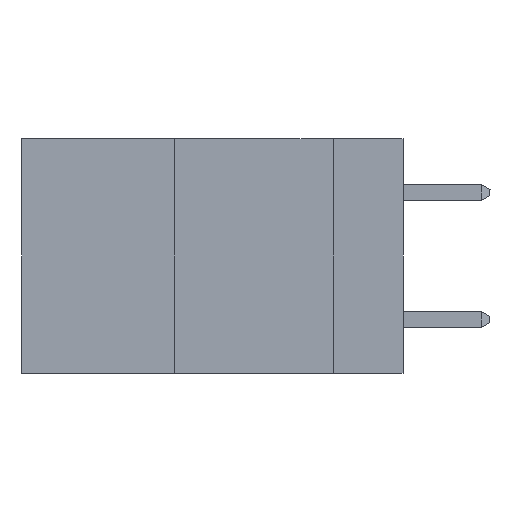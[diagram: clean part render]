
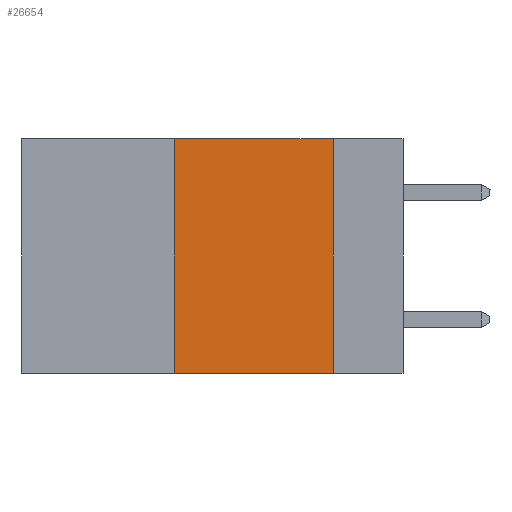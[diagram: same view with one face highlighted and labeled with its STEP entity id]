
A CAD part, left-side view. The second image highlights one B-rep face of the part: STEP entity #26654.
In plain terms, the highlighted planar face has unit normal (-1, 0, 0).
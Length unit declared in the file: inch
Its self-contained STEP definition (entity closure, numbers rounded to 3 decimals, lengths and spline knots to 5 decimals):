
#733 = VERTEX_POINT ( 'NONE', #2641 ) ;
#1047 = VECTOR ( 'NONE', #27830, 39.37008 ) ;
#1316 = VECTOR ( 'NONE', #24645, 39.37008 ) ;
#1868 = EDGE_LOOP ( 'NONE', ( #24799, #25606, #3925, #4275 ) ) ;
#2158 = EDGE_CURVE ( 'NONE', #22826, #16824, #6789, .T. ) ;
#2383 = LINE ( 'NONE', #14751, #27492 ) ;
#2428 = CARTESIAN_POINT ( 'NONE',  ( 0., 0.36, 0. ) ) ;
#2641 = CARTESIAN_POINT ( 'NONE',  ( 0., 0.11, -0.37 ) ) ;
#3925 = ORIENTED_EDGE ( 'NONE', *, *, #2158, .F. ) ;
#3987 = DIRECTION ( 'NONE',  ( 0., -1., 0. ) ) ;
#4230 = PLANE ( 'NONE',  #8082 ) ;
#4275 = ORIENTED_EDGE ( 'NONE', *, *, #17643, .T. ) ;
#4568 = DIRECTION ( 'NONE',  ( 0., 0., -1. ) ) ;
#4809 = CARTESIAN_POINT ( 'NONE',  ( 0., 0.11, 0. ) ) ;
#6434 = VERTEX_POINT ( 'NONE', #4809 ) ;
#6624 = CARTESIAN_POINT ( 'NONE',  ( 0., 0.11, 0. ) ) ;
#6789 = LINE ( 'NONE', #2428, #1047 ) ;
#7652 = EDGE_CURVE ( 'NONE', #16824, #6434, #24380, .T. ) ;
#8082 = AXIS2_PLACEMENT_3D ( 'NONE', #21525, #8178, #21116 ) ;
#8178 = DIRECTION ( 'NONE',  ( 1., 0., 0. ) ) ;
#9931 = CARTESIAN_POINT ( 'NONE',  ( 0., 0.36, 0. ) ) ;
#11868 = VECTOR ( 'NONE', #4568, 39.37008 ) ;
#14074 = CARTESIAN_POINT ( 'NONE',  ( 0., 0.6, 0. ) ) ;
#14751 = CARTESIAN_POINT ( 'NONE',  ( 0., 0.6, -0.37 ) ) ;
#16824 = VERTEX_POINT ( 'NONE', #9931 ) ;
#17123 = EDGE_CURVE ( 'NONE', #6434, #733, #17613, .T. ) ;
#17613 = LINE ( 'NONE', #6624, #11868 ) ;
#17643 = EDGE_CURVE ( 'NONE', #22826, #733, #2383, .T. ) ;
#21116 = DIRECTION ( 'NONE',  ( 0., 0., -1. ) ) ;
#21525 = CARTESIAN_POINT ( 'NONE',  ( 0., 0.6, 0. ) ) ;
#22826 = VERTEX_POINT ( 'NONE', #26526 ) ;
#24380 = LINE ( 'NONE', #14074, #1316 ) ;
#24645 = DIRECTION ( 'NONE',  ( 0., -1., 0. ) ) ;
#24799 = ORIENTED_EDGE ( 'NONE', *, *, #17123, .F. ) ;
#25606 = ORIENTED_EDGE ( 'NONE', *, *, #7652, .F. ) ;
#26526 = CARTESIAN_POINT ( 'NONE',  ( 0., 0.36, -0.37 ) ) ;
#26654 = ADVANCED_FACE ( 'NONE', ( #26952 ), #4230, .F. ) ;
#26952 = FACE_OUTER_BOUND ( 'NONE', #1868, .T. ) ;
#27492 = VECTOR ( 'NONE', #3987, 39.37008 ) ;
#27830 = DIRECTION ( 'NONE',  ( 0., 0., 1. ) ) ;
